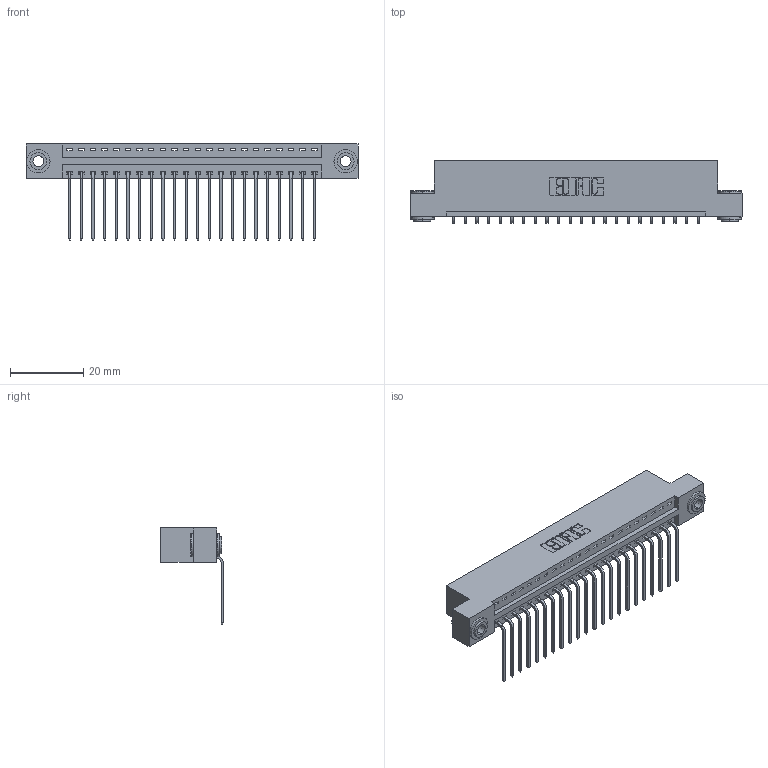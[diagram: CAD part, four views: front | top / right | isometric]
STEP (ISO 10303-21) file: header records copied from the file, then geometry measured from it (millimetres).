
FILE_DESCRIPTION (( 'STEP AP203' ), '1' );
FILE_NAME ('346-022-559-103.STEP', '2022-05-05T20:15:05', ( '' ), ( '' ), 'SwSTEP 2.0', 'SolidWorks 2020', '' );
FILE_SCHEMA (( 'CONFIG_CONTROL_DESIGN' ));
Length unit declared in the file: inch
Products named in the file (4): 346 Part_Flush Mounting Lugs - 0.156 Dia-TH; 346-022-559-103; 345-250-002_345-250-002-102; 345-292-001_558 559 Tail - 1
Assembly tree (25 placements, depth 2):
  346-022-559-103
    346 Part_Flush Mounting Lugs - 0.156 Dia-TH
    345-292-001_558 559 Tail - 1  x22
    345-250-002_345-250-002-102  x2
Bounding box: 90.42 x 17.08 x 26.16 mm (x, y, z)
Volume: 8592.4 mm3; surface area: 11212.3 mm2
Topology: 25 solids, 25 shells, 1494 faces, 4445 edges, 2930 vertices
Faces by surface type: plane 1024, cylinder 462, cone 8
Entity records: 17496 total; most frequent: CARTESIAN_POINT 2987, ORIENTED_EDGE 2934, DIRECTION 2689, EDGE_CURVE 1467, VECTOR 1223, LINE 1223, VERTEX_POINT 974, AXIS2_PLACEMENT_3D 733
